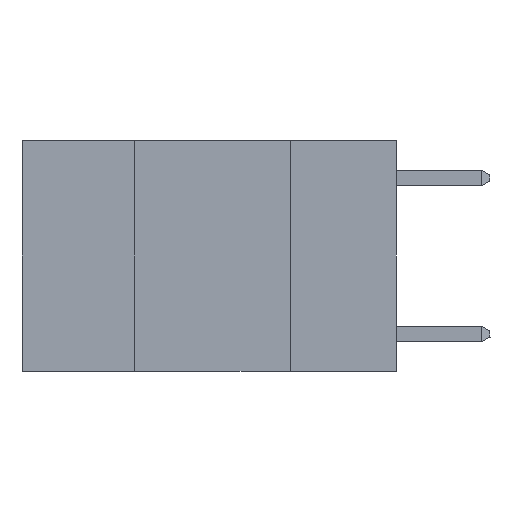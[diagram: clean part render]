
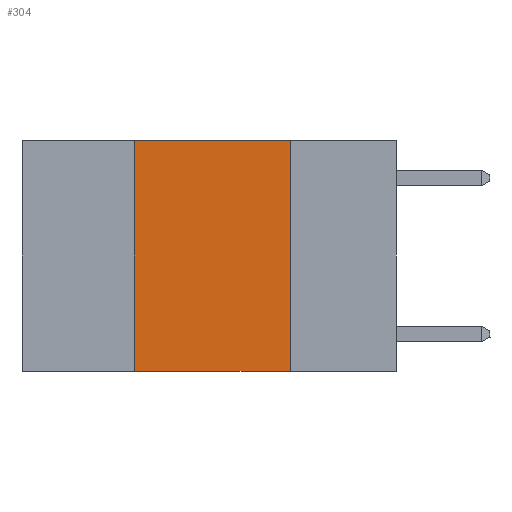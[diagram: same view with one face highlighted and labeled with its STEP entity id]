
A CAD part, left-side view. The second image highlights one B-rep face of the part: STEP entity #304.
In plain terms, the highlighted planar face has unit normal (-1, 0, 0).
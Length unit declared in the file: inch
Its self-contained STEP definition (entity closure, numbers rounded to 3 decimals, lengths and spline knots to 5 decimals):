
#304 = ADVANCED_FACE ( 'NONE', ( #6854 ), #11064, .F. ) ;
#815 = EDGE_LOOP ( 'NONE', ( #1309, #8204, #986, #10262 ) ) ;
#986 = ORIENTED_EDGE ( 'NONE', *, *, #8098, .F. ) ;
#1309 = ORIENTED_EDGE ( 'NONE', *, *, #1449, .F. ) ;
#1449 = EDGE_CURVE ( 'NONE', #11092, #8309, #11580, .T. ) ;
#2066 = DIRECTION ( 'NONE',  ( 0., -1., 0. ) ) ;
#2091 = LINE ( 'NONE', #10578, #6502 ) ;
#2176 = CARTESIAN_POINT ( 'NONE',  ( 0., 0.6, -0.37 ) ) ;
#2427 = CARTESIAN_POINT ( 'NONE',  ( 0., 0.6, 0. ) ) ;
#2617 = VECTOR ( 'NONE', #2066, 39.37008 ) ;
#2766 = CARTESIAN_POINT ( 'NONE',  ( 0., 0.17, -0.37 ) ) ;
#3315 = DIRECTION ( 'NONE',  ( 0., -1., 0. ) ) ;
#3488 = VERTEX_POINT ( 'NONE', #5800 ) ;
#3619 = EDGE_CURVE ( 'NONE', #3997, #8309, #4666, .T. ) ;
#3932 = DIRECTION ( 'NONE',  ( 0., 0., -1. ) ) ;
#3997 = VERTEX_POINT ( 'NONE', #9779 ) ;
#4145 = DIRECTION ( 'NONE',  ( 1., 0., 0. ) ) ;
#4188 = LINE ( 'NONE', #2427, #8710 ) ;
#4436 = VECTOR ( 'NONE', #4941, 39.37008 ) ;
#4666 = LINE ( 'NONE', #2176, #2617 ) ;
#4941 = DIRECTION ( 'NONE',  ( 0., 0., -1. ) ) ;
#5084 = EDGE_CURVE ( 'NONE', #3488, #11092, #4188, .T. ) ;
#5800 = CARTESIAN_POINT ( 'NONE',  ( 0., 0.42, 0. ) ) ;
#6452 = AXIS2_PLACEMENT_3D ( 'NONE', #10999, #4145, #3932 ) ;
#6502 = VECTOR ( 'NONE', #11437, 39.37008 ) ;
#6854 = FACE_OUTER_BOUND ( 'NONE', #815, .T. ) ;
#7502 = CARTESIAN_POINT ( 'NONE',  ( 0., 0.17, 0. ) ) ;
#8098 = EDGE_CURVE ( 'NONE', #3997, #3488, #2091, .T. ) ;
#8204 = ORIENTED_EDGE ( 'NONE', *, *, #5084, .F. ) ;
#8309 = VERTEX_POINT ( 'NONE', #2766 ) ;
#8710 = VECTOR ( 'NONE', #3315, 39.37008 ) ;
#9779 = CARTESIAN_POINT ( 'NONE',  ( 0., 0.42, -0.37 ) ) ;
#10262 = ORIENTED_EDGE ( 'NONE', *, *, #3619, .T. ) ;
#10578 = CARTESIAN_POINT ( 'NONE',  ( 0., 0.42, 0. ) ) ;
#10999 = CARTESIAN_POINT ( 'NONE',  ( 0., 0.6, 0. ) ) ;
#11064 = PLANE ( 'NONE',  #6452 ) ;
#11092 = VERTEX_POINT ( 'NONE', #7502 ) ;
#11151 = CARTESIAN_POINT ( 'NONE',  ( 0., 0.17, 0. ) ) ;
#11437 = DIRECTION ( 'NONE',  ( 0., 0., 1. ) ) ;
#11580 = LINE ( 'NONE', #11151, #4436 ) ;
